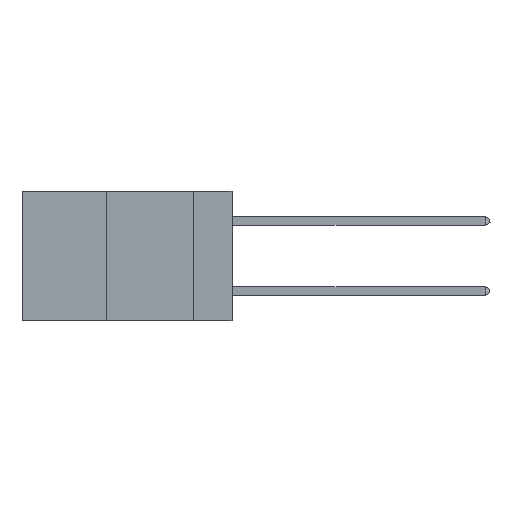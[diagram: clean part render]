
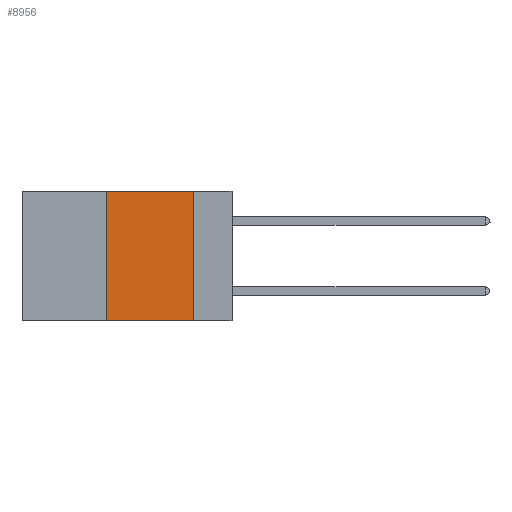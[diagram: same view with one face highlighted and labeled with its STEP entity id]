
A CAD part, left-side view. The second image highlights one B-rep face of the part: STEP entity #8956.
In plain terms, the highlighted planar face has unit normal (-1, 0, 0).
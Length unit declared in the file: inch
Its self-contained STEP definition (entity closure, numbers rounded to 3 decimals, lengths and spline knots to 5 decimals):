
#52 = LINE ( 'NONE', #7687, #12855 ) ;
#138 = EDGE_LOOP ( 'NONE', ( #6098, #6244, #6410, #6497 ) ) ;
#188 = VECTOR ( 'NONE', #12995, 39.37008 ) ;
#1165 = PLANE ( 'NONE',  #6659 ) ;
#1482 = LINE ( 'NONE', #10780, #7713 ) ;
#2460 = DIRECTION ( 'NONE',  ( 1., 0., 0. ) ) ;
#4066 = DIRECTION ( 'NONE',  ( 0., -1., 0. ) ) ;
#4411 = EDGE_CURVE ( 'NONE', #10578, #9842, #1482, .T. ) ;
#4464 = VERTEX_POINT ( 'NONE', #4782 ) ;
#4704 = EDGE_CURVE ( 'NONE', #10578, #15144, #52, .T. ) ;
#4770 = VECTOR ( 'NONE', #4066, 39.37008 ) ;
#4782 = CARTESIAN_POINT ( 'NONE',  ( 0., 0.11, 0. ) ) ;
#6098 = ORIENTED_EDGE ( 'NONE', *, *, #15103, .F. ) ;
#6244 = ORIENTED_EDGE ( 'NONE', *, *, #6369, .F. ) ;
#6369 = EDGE_CURVE ( 'NONE', #9842, #4464, #14148, .T. ) ;
#6410 = ORIENTED_EDGE ( 'NONE', *, *, #4411, .F. ) ;
#6497 = ORIENTED_EDGE ( 'NONE', *, *, #4704, .T. ) ;
#6659 = AXIS2_PLACEMENT_3D ( 'NONE', #8638, #2460, #11055 ) ;
#6926 = CARTESIAN_POINT ( 'NONE',  ( 0., 0.11, 0. ) ) ;
#6929 = CARTESIAN_POINT ( 'NONE',  ( 0., 0.36, -0.37 ) ) ;
#7631 = LINE ( 'NONE', #6926, #188 ) ;
#7687 = CARTESIAN_POINT ( 'NONE',  ( 0., 0.6, -0.37 ) ) ;
#7713 = VECTOR ( 'NONE', #9565, 39.37008 ) ;
#8638 = CARTESIAN_POINT ( 'NONE',  ( 0., 0.6, 0. ) ) ;
#8956 = ADVANCED_FACE ( 'NONE', ( #12336 ), #1165, .F. ) ;
#9565 = DIRECTION ( 'NONE',  ( 0., 0., 1. ) ) ;
#9842 = VERTEX_POINT ( 'NONE', #15201 ) ;
#10146 = DIRECTION ( 'NONE',  ( 0., -1., 0. ) ) ;
#10578 = VERTEX_POINT ( 'NONE', #6929 ) ;
#10780 = CARTESIAN_POINT ( 'NONE',  ( 0., 0.36, 0. ) ) ;
#11055 = DIRECTION ( 'NONE',  ( 0., 0., -1. ) ) ;
#11392 = CARTESIAN_POINT ( 'NONE',  ( 0., 0.6, 0. ) ) ;
#12336 = FACE_OUTER_BOUND ( 'NONE', #138, .T. ) ;
#12855 = VECTOR ( 'NONE', #10146, 39.37008 ) ;
#12995 = DIRECTION ( 'NONE',  ( 0., 0., -1. ) ) ;
#14148 = LINE ( 'NONE', #11392, #4770 ) ;
#14314 = CARTESIAN_POINT ( 'NONE',  ( 0., 0.11, -0.37 ) ) ;
#15103 = EDGE_CURVE ( 'NONE', #4464, #15144, #7631, .T. ) ;
#15144 = VERTEX_POINT ( 'NONE', #14314 ) ;
#15201 = CARTESIAN_POINT ( 'NONE',  ( 0., 0.36, 0. ) ) ;
